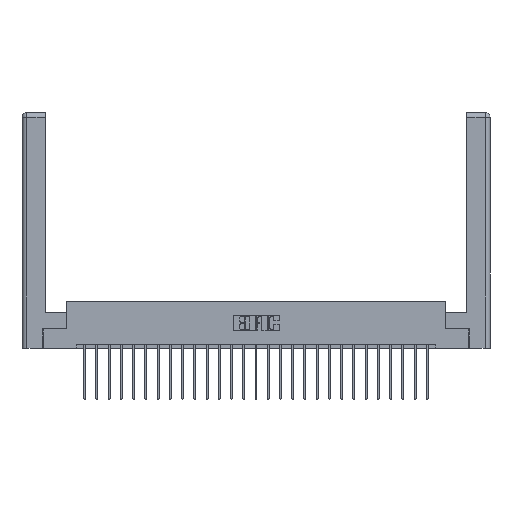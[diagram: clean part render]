
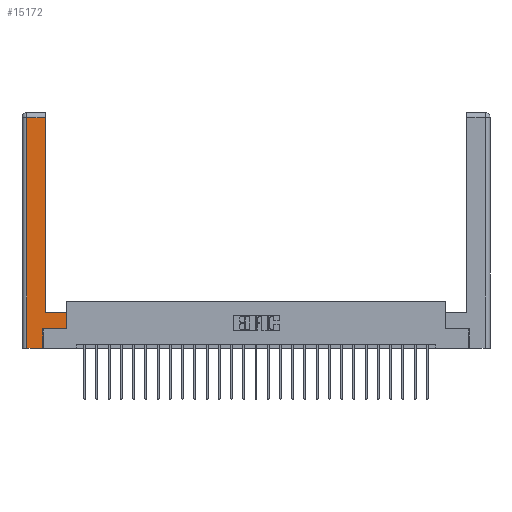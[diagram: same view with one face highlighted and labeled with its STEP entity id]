
A CAD part, top view. The second image highlights one B-rep face of the part: STEP entity #15172.
In plain terms, the highlighted planar face has unit normal (0, 0, 1).
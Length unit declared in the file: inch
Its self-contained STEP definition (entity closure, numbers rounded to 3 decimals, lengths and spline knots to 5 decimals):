
#104 = LINE ( 'NONE', #9397, #2003 ) ;
#117 = DIRECTION ( 'NONE',  ( 1., 0., 0. ) ) ;
#470 = VECTOR ( 'NONE', #21550, 39.37008 ) ;
#2003 = VECTOR ( 'NONE', #22041, 39.37008 ) ;
#2096 = CARTESIAN_POINT ( 'NONE',  ( 0.265, 0.245, 0. ) ) ;
#2713 = VERTEX_POINT ( 'NONE', #23744 ) ;
#3101 = AXIS2_PLACEMENT_3D ( 'NONE', #7047, #8869, #15332 ) ;
#3133 = CARTESIAN_POINT ( 'NONE',  ( 0.265, 0., 0. ) ) ;
#3873 = ORIENTED_EDGE ( 'NONE', *, *, #20317, .T. ) ;
#4346 = DIRECTION ( 'NONE',  ( -1., 0., 0. ) ) ;
#4764 = ORIENTED_EDGE ( 'NONE', *, *, #11614, .T. ) ;
#5929 = VECTOR ( 'NONE', #117, 39.37008 ) ;
#6499 = DIRECTION ( 'NONE',  ( 0., -1., 0. ) ) ;
#7047 = CARTESIAN_POINT ( 'NONE',  ( 0., 0., 0. ) ) ;
#7432 = DIRECTION ( 'NONE',  ( 1., 0., 0. ) ) ;
#7581 = LINE ( 'NONE', #8225, #19330 ) ;
#7879 = EDGE_CURVE ( 'NONE', #9051, #21931, #11118, .T. ) ;
#8225 = CARTESIAN_POINT ( 'NONE',  ( 0.295, 3., 0. ) ) ;
#8339 = CARTESIAN_POINT ( 'NONE',  ( 0.0615, 2.94, 0. ) ) ;
#8403 = DIRECTION ( 'NONE',  ( 0., 1., 0. ) ) ;
#8557 = ORIENTED_EDGE ( 'NONE', *, *, #26017, .T. ) ;
#8635 = EDGE_LOOP ( 'NONE', ( #3873, #11482, #12300, #4764, #19582, #14501, #12499, #8557 ) ) ;
#8856 = VERTEX_POINT ( 'NONE', #3133 ) ;
#8869 = DIRECTION ( 'NONE',  ( 0., 0., -1. ) ) ;
#9051 = VERTEX_POINT ( 'NONE', #13868 ) ;
#9397 = CARTESIAN_POINT ( 'NONE',  ( 0.295, 0.45, 0. ) ) ;
#9436 = LINE ( 'NONE', #18778, #17222 ) ;
#10601 = CARTESIAN_POINT ( 'NONE',  ( 0.565, 0.245, 0. ) ) ;
#11118 = LINE ( 'NONE', #10601, #5929 ) ;
#11482 = ORIENTED_EDGE ( 'NONE', *, *, #17632, .T. ) ;
#11614 = EDGE_CURVE ( 'NONE', #23717, #8856, #24406, .T. ) ;
#11933 = EDGE_CURVE ( 'NONE', #8856, #9051, #22456, .T. ) ;
#12300 = ORIENTED_EDGE ( 'NONE', *, *, #17517, .T. ) ;
#12499 = ORIENTED_EDGE ( 'NONE', *, *, #26584, .T. ) ;
#13868 = CARTESIAN_POINT ( 'NONE',  ( 0.265, 0.245, 0. ) ) ;
#14037 = VECTOR ( 'NONE', #7432, 39.37008 ) ;
#14501 = ORIENTED_EDGE ( 'NONE', *, *, #7879, .T. ) ;
#14948 = VECTOR ( 'NONE', #4346, 39.37008 ) ;
#15172 = ADVANCED_FACE ( 'NONE', ( #19683 ), #21520, .F. ) ;
#15332 = DIRECTION ( 'NONE',  ( -1., 0., 0. ) ) ;
#17011 = LINE ( 'NONE', #25692, #470 ) ;
#17222 = VECTOR ( 'NONE', #6499, 39.37008 ) ;
#17517 = EDGE_CURVE ( 'NONE', #20788, #23717, #9436, .T. ) ;
#17632 = EDGE_CURVE ( 'NONE', #25541, #20788, #20496, .T. ) ;
#17703 = VERTEX_POINT ( 'NONE', #23294 ) ;
#17835 = CARTESIAN_POINT ( 'NONE',  ( 0.0615, 2.94, 0. ) ) ;
#18226 = CARTESIAN_POINT ( 'NONE',  ( 0.0615, 0., 0. ) ) ;
#18778 = CARTESIAN_POINT ( 'NONE',  ( 0.0615, 0., 0. ) ) ;
#19298 = CARTESIAN_POINT ( 'NONE',  ( 0.565, 0.245, 0. ) ) ;
#19330 = VECTOR ( 'NONE', #8403, 39.37008 ) ;
#19582 = ORIENTED_EDGE ( 'NONE', *, *, #11933, .T. ) ;
#19683 = FACE_OUTER_BOUND ( 'NONE', #8635, .T. ) ;
#20317 = EDGE_CURVE ( 'NONE', #17703, #25541, #7581, .T. ) ;
#20496 = LINE ( 'NONE', #8339, #14948 ) ;
#20788 = VERTEX_POINT ( 'NONE', #17835 ) ;
#21520 = PLANE ( 'NONE',  #3101 ) ;
#21550 = DIRECTION ( 'NONE',  ( 0., 1., 0. ) ) ;
#21931 = VERTEX_POINT ( 'NONE', #19298 ) ;
#22041 = DIRECTION ( 'NONE',  ( -1., 0., 0. ) ) ;
#22456 = LINE ( 'NONE', #2096, #23078 ) ;
#22770 = CARTESIAN_POINT ( 'NONE',  ( 0.295, 2.94, 0. ) ) ;
#23078 = VECTOR ( 'NONE', #25039, 39.37008 ) ;
#23294 = CARTESIAN_POINT ( 'NONE',  ( 0.295, 0.45, 0. ) ) ;
#23717 = VERTEX_POINT ( 'NONE', #18226 ) ;
#23744 = CARTESIAN_POINT ( 'NONE',  ( 0.565, 0.45, 0. ) ) ;
#24141 = CARTESIAN_POINT ( 'NONE',  ( 0.265, 0., 0. ) ) ;
#24406 = LINE ( 'NONE', #24141, #14037 ) ;
#25039 = DIRECTION ( 'NONE',  ( 0., 1., 0. ) ) ;
#25541 = VERTEX_POINT ( 'NONE', #22770 ) ;
#25692 = CARTESIAN_POINT ( 'NONE',  ( 0.565, 0.45, 0. ) ) ;
#26017 = EDGE_CURVE ( 'NONE', #2713, #17703, #104, .T. ) ;
#26584 = EDGE_CURVE ( 'NONE', #21931, #2713, #17011, .T. ) ;
